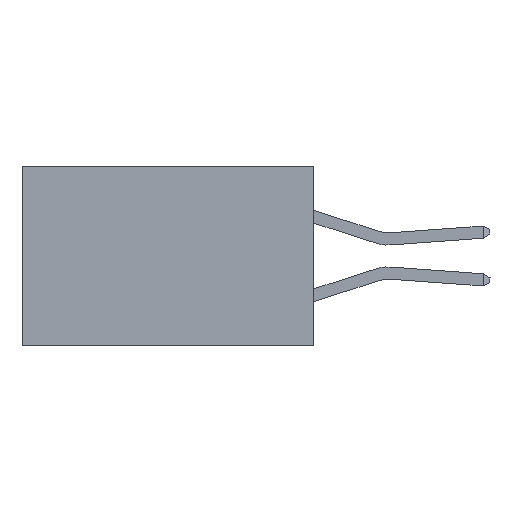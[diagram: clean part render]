
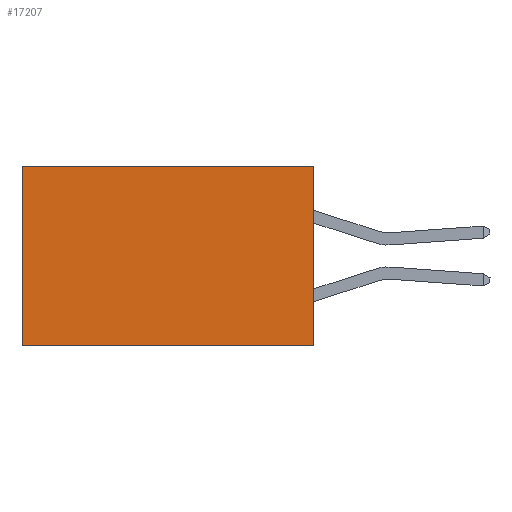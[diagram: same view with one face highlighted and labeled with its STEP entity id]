
A CAD part, left-side view. The second image highlights one B-rep face of the part: STEP entity #17207.
In plain terms, the highlighted planar face has unit normal (-1, 0, 0).
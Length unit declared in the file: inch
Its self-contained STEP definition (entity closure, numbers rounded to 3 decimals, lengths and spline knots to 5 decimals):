
#571 = DIRECTION ( 'NONE',  ( 1., 0., 0. ) ) ;
#617 = CARTESIAN_POINT ( 'NONE',  ( 0.2875, 0., 0. ) ) ;
#1414 = ORIENTED_EDGE ( 'NONE', *, *, #18622, .T. ) ;
#1551 = CARTESIAN_POINT ( 'NONE',  ( 0.2875, 0., -0.37 ) ) ;
#1900 = VECTOR ( 'NONE', #10684, 39.37008 ) ;
#1971 = VERTEX_POINT ( 'NONE', #20139 ) ;
#2403 = LINE ( 'NONE', #20649, #1900 ) ;
#2603 = AXIS2_PLACEMENT_3D ( 'NONE', #10056, #571, #11659 ) ;
#5215 = CARTESIAN_POINT ( 'NONE',  ( 0.2875, 0., 0. ) ) ;
#5571 = CARTESIAN_POINT ( 'NONE',  ( 0.2875, 0., -0.37 ) ) ;
#6054 = LINE ( 'NONE', #5215, #18519 ) ;
#6310 = LINE ( 'NONE', #1551, #14874 ) ;
#7444 = VECTOR ( 'NONE', #11745, 39.37008 ) ;
#7596 = FACE_OUTER_BOUND ( 'NONE', #15596, .T. ) ;
#7601 = EDGE_CURVE ( 'NONE', #1971, #16755, #2403, .T. ) ;
#8955 = CARTESIAN_POINT ( 'NONE',  ( 0.2875, 0.6, -0.37 ) ) ;
#10056 = CARTESIAN_POINT ( 'NONE',  ( 0.2875, 0., 0. ) ) ;
#10328 = EDGE_CURVE ( 'NONE', #16006, #20040, #16654, .T. ) ;
#10684 = DIRECTION ( 'NONE',  ( 0., 0., -1. ) ) ;
#11301 = ORIENTED_EDGE ( 'NONE', *, *, #18376, .F. ) ;
#11592 = PLANE ( 'NONE',  #2603 ) ;
#11659 = DIRECTION ( 'NONE',  ( 0., 0., -1. ) ) ;
#11745 = DIRECTION ( 'NONE',  ( 0., 0., -1. ) ) ;
#12619 = DIRECTION ( 'NONE',  ( 0., 1., 0. ) ) ;
#13984 = ORIENTED_EDGE ( 'NONE', *, *, #7601, .T. ) ;
#14824 = DIRECTION ( 'NONE',  ( 0., 1., 0. ) ) ;
#14874 = VECTOR ( 'NONE', #12619, 39.37008 ) ;
#15596 = EDGE_LOOP ( 'NONE', ( #13984, #11301, #19233, #1414 ) ) ;
#16006 = VERTEX_POINT ( 'NONE', #617 ) ;
#16654 = LINE ( 'NONE', #19942, #7444 ) ;
#16755 = VERTEX_POINT ( 'NONE', #8955 ) ;
#17207 = ADVANCED_FACE ( 'NONE', ( #7596 ), #11592, .F. ) ;
#18376 = EDGE_CURVE ( 'NONE', #20040, #16755, #6310, .T. ) ;
#18519 = VECTOR ( 'NONE', #14824, 39.37008 ) ;
#18622 = EDGE_CURVE ( 'NONE', #16006, #1971, #6054, .T. ) ;
#19233 = ORIENTED_EDGE ( 'NONE', *, *, #10328, .F. ) ;
#19942 = CARTESIAN_POINT ( 'NONE',  ( 0.2875, 0., 0. ) ) ;
#20040 = VERTEX_POINT ( 'NONE', #5571 ) ;
#20139 = CARTESIAN_POINT ( 'NONE',  ( 0.2875, 0.6, 0. ) ) ;
#20649 = CARTESIAN_POINT ( 'NONE',  ( 0.2875, 0.6, 0. ) ) ;
